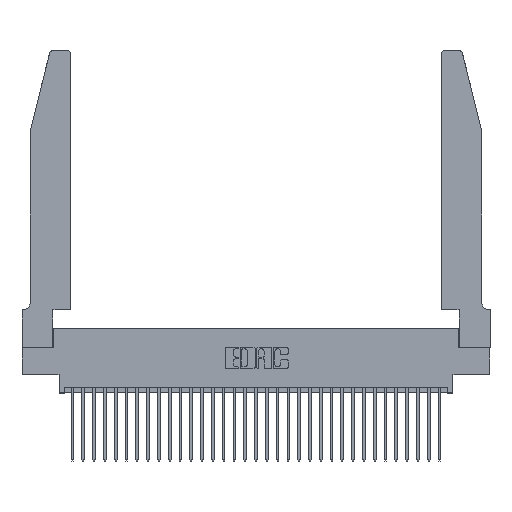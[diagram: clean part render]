
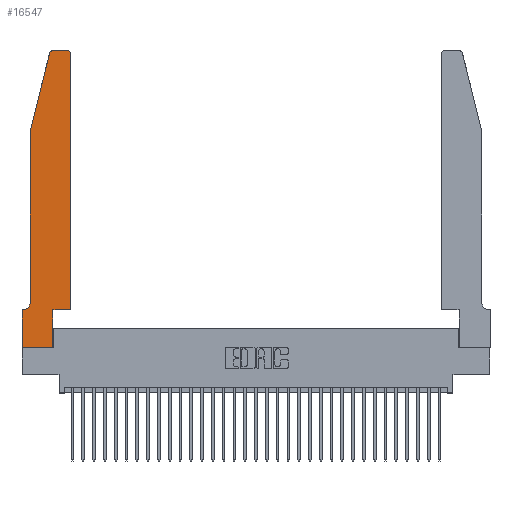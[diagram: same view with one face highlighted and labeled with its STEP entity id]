
A CAD part, top view. The second image highlights one B-rep face of the part: STEP entity #16547.
In plain terms, the highlighted planar face has unit normal (0, 0, 1).
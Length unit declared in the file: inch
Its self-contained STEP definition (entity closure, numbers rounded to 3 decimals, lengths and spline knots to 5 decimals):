
#813 = DIRECTION ( 'NONE',  ( 0., -1., 0. ) ) ;
#878 = CARTESIAN_POINT ( 'NONE',  ( 0.2865, 0.35, 0.37 ) ) ;
#1207 = AXIS2_PLACEMENT_3D ( 'NONE', #14148, #31943, #16681 ) ;
#1760 = VECTOR ( 'NONE', #32668, 39.37008 ) ;
#1921 = VERTEX_POINT ( 'NONE', #11073 ) ;
#1979 = AXIS2_PLACEMENT_3D ( 'NONE', #20696, #5281, #23230 ) ;
#2362 = CARTESIAN_POINT ( 'NONE',  ( 0.0755, 0.35, 0.37 ) ) ;
#2518 = VECTOR ( 'NONE', #28726, 39.37008 ) ;
#2587 = LINE ( 'NONE', #27546, #1760 ) ;
#2702 = CARTESIAN_POINT ( 'NONE',  ( 0., 0., 0.37 ) ) ;
#3361 = CARTESIAN_POINT ( 'NONE',  ( 0., 0., 0.37 ) ) ;
#3857 = ORIENTED_EDGE ( 'NONE', *, *, #23482, .T. ) ;
#4742 = VERTEX_POINT ( 'NONE', #878 ) ;
#4816 = CARTESIAN_POINT ( 'NONE',  ( 0., 0., 0.37 ) ) ;
#5028 = VECTOR ( 'NONE', #7811, 39.37008 ) ;
#5113 = EDGE_CURVE ( 'NONE', #18252, #1921, #32019, .T. ) ;
#5281 = DIRECTION ( 'NONE',  ( 0., 0., -1. ) ) ;
#5404 = CIRCLE ( 'NONE', #9848, 0.03 ) ;
#5429 = DIRECTION ( 'NONE',  ( 0., 0., 1. ) ) ;
#5750 = EDGE_LOOP ( 'NONE', ( #21604, #10307, #29252, #15406, #27649, #21780, #27884, #14584, #3857, #28914, #32322, #11467 ) ) ;
#5768 = DIRECTION ( 'NONE',  ( 0., 1., 0. ) ) ;
#5842 = LINE ( 'NONE', #15907, #5028 ) ;
#6312 = DIRECTION ( 'NONE',  ( 1., 0., 0. ) ) ;
#6433 = VECTOR ( 'NONE', #18829, 39.37008 ) ;
#7139 = CIRCLE ( 'NONE', #1979, 0.07 ) ;
#7418 = DIRECTION ( 'NONE',  ( 1., 0., 0. ) ) ;
#7811 = DIRECTION ( 'NONE',  ( 0., 1., 0. ) ) ;
#8210 = VECTOR ( 'NONE', #813, 39.37008 ) ;
#8609 = VERTEX_POINT ( 'NONE', #20761 ) ;
#8760 = CARTESIAN_POINT ( 'NONE',  ( 0.0755, 0.42, 0.37 ) ) ;
#8804 = LINE ( 'NONE', #14007, #21606 ) ;
#9197 = EDGE_CURVE ( 'NONE', #11181, #30884, #23069, .T. ) ;
#9830 = LINE ( 'NONE', #18953, #8210 ) ;
#9848 = AXIS2_PLACEMENT_3D ( 'NONE', #20848, #5429, #23370 ) ;
#10081 = FACE_OUTER_BOUND ( 'NONE', #5750, .T. ) ;
#10307 = ORIENTED_EDGE ( 'NONE', *, *, #17430, .T. ) ;
#10572 = EDGE_CURVE ( 'NONE', #26296, #20431, #7139, .T. ) ;
#11073 = CARTESIAN_POINT ( 'NONE',  ( 0.2865, 0., 0.37 ) ) ;
#11181 = VERTEX_POINT ( 'NONE', #20893 ) ;
#11467 = ORIENTED_EDGE ( 'NONE', *, *, #24895, .T. ) ;
#13469 = CARTESIAN_POINT ( 'NONE',  ( 0.2865, 0.35, 0.37 ) ) ;
#13632 = LINE ( 'NONE', #13469, #33137 ) ;
#13900 = LINE ( 'NONE', #2362, #27417 ) ;
#13901 = AXIS2_PLACEMENT_3D ( 'NONE', #30561, #15332, #33114 ) ;
#14007 = CARTESIAN_POINT ( 'NONE',  ( 0.4505, 0.35, 0.37 ) ) ;
#14148 = CARTESIAN_POINT ( 'NONE',  ( 0., 0.35, 0.37 ) ) ;
#14584 = ORIENTED_EDGE ( 'NONE', *, *, #5113, .T. ) ;
#15332 = DIRECTION ( 'NONE',  ( 0., 0., 1. ) ) ;
#15406 = ORIENTED_EDGE ( 'NONE', *, *, #20255, .T. ) ;
#15428 = VERTEX_POINT ( 'NONE', #19218 ) ;
#15723 = CARTESIAN_POINT ( 'NONE',  ( 0.284, 2.75, 0.37 ) ) ;
#15844 = CARTESIAN_POINT ( 'NONE',  ( 0.25487, 2.72718, 0.37 ) ) ;
#15907 = CARTESIAN_POINT ( 'NONE',  ( 0.4505, 0.35, 0.37 ) ) ;
#16451 = EDGE_CURVE ( 'NONE', #18046, #18252, #19289, .T. ) ;
#16547 = ADVANCED_FACE ( 'NONE', ( #10081 ), #29381, .T. ) ;
#16681 = DIRECTION ( 'NONE',  ( 1., 0., 0. ) ) ;
#17430 = EDGE_CURVE ( 'NONE', #30884, #26132, #29557, .T. ) ;
#18046 = VERTEX_POINT ( 'NONE', #22545 ) ;
#18252 = VERTEX_POINT ( 'NONE', #2702 ) ;
#18490 = VECTOR ( 'NONE', #7418, 39.37008 ) ;
#18829 = DIRECTION ( 'NONE',  ( 0., -1., 0. ) ) ;
#18953 = CARTESIAN_POINT ( 'NONE',  ( 0.0755, 2., 0.37 ) ) ;
#19000 = EDGE_CURVE ( 'NONE', #28750, #15428, #5842, .T. ) ;
#19218 = CARTESIAN_POINT ( 'NONE',  ( 0.4505, 2.72, 0.37 ) ) ;
#19289 = LINE ( 'NONE', #3361, #6433 ) ;
#19620 = CARTESIAN_POINT ( 'NONE',  ( 0.0055, 0.35, 0.37 ) ) ;
#20255 = EDGE_CURVE ( 'NONE', #8609, #26296, #9830, .T. ) ;
#20431 = VERTEX_POINT ( 'NONE', #19620 ) ;
#20433 = DIRECTION ( 'NONE',  ( -1., 0., 0. ) ) ;
#20696 = CARTESIAN_POINT ( 'NONE',  ( 0.0055, 0.42, 0.37 ) ) ;
#20761 = CARTESIAN_POINT ( 'NONE',  ( 0.0755, 2., 0.37 ) ) ;
#20848 = CARTESIAN_POINT ( 'NONE',  ( 0.4205, 2.72, 0.37 ) ) ;
#20893 = CARTESIAN_POINT ( 'NONE',  ( 0.4205, 2.75, 0.37 ) ) ;
#21604 = ORIENTED_EDGE ( 'NONE', *, *, #9197, .T. ) ;
#21606 = VECTOR ( 'NONE', #6312, 39.37008 ) ;
#21780 = ORIENTED_EDGE ( 'NONE', *, *, #25995, .T. ) ;
#22545 = CARTESIAN_POINT ( 'NONE',  ( 0., 0.35, 0.37 ) ) ;
#23069 = LINE ( 'NONE', #26146, #2518 ) ;
#23230 = DIRECTION ( 'NONE',  ( -1., 0., 0. ) ) ;
#23370 = DIRECTION ( 'NONE',  ( 1., 0., 0. ) ) ;
#23482 = EDGE_CURVE ( 'NONE', #1921, #4742, #13632, .T. ) ;
#24895 = EDGE_CURVE ( 'NONE', #15428, #11181, #5404, .T. ) ;
#25995 = EDGE_CURVE ( 'NONE', #20431, #18046, #13900, .T. ) ;
#26132 = VERTEX_POINT ( 'NONE', #15844 ) ;
#26146 = CARTESIAN_POINT ( 'NONE',  ( 0.2605, 2.75, 0.37 ) ) ;
#26296 = VERTEX_POINT ( 'NONE', #8760 ) ;
#27341 = CARTESIAN_POINT ( 'NONE',  ( 0.4505, 0.35, 0.37 ) ) ;
#27417 = VECTOR ( 'NONE', #20433, 39.37008 ) ;
#27546 = CARTESIAN_POINT ( 'NONE',  ( 0.0755, 2., 0.37 ) ) ;
#27649 = ORIENTED_EDGE ( 'NONE', *, *, #10572, .T. ) ;
#27884 = ORIENTED_EDGE ( 'NONE', *, *, #16451, .T. ) ;
#28726 = DIRECTION ( 'NONE',  ( -1., 0., 0. ) ) ;
#28750 = VERTEX_POINT ( 'NONE', #27341 ) ;
#28914 = ORIENTED_EDGE ( 'NONE', *, *, #31587, .T. ) ;
#29252 = ORIENTED_EDGE ( 'NONE', *, *, #32471, .T. ) ;
#29381 = PLANE ( 'NONE',  #1207 ) ;
#29557 = CIRCLE ( 'NONE', #13901, 0.03 ) ;
#30561 = CARTESIAN_POINT ( 'NONE',  ( 0.284, 2.72, 0.37 ) ) ;
#30884 = VERTEX_POINT ( 'NONE', #15723 ) ;
#31587 = EDGE_CURVE ( 'NONE', #4742, #28750, #8804, .T. ) ;
#31943 = DIRECTION ( 'NONE',  ( 0., 0., 1. ) ) ;
#32019 = LINE ( 'NONE', #4816, #18490 ) ;
#32322 = ORIENTED_EDGE ( 'NONE', *, *, #19000, .T. ) ;
#32471 = EDGE_CURVE ( 'NONE', #26132, #8609, #2587, .T. ) ;
#32668 = DIRECTION ( 'NONE',  ( -0.239, -0.971, 0. ) ) ;
#33114 = DIRECTION ( 'NONE',  ( 1., 0., 0. ) ) ;
#33137 = VECTOR ( 'NONE', #5768, 39.37008 ) ;
